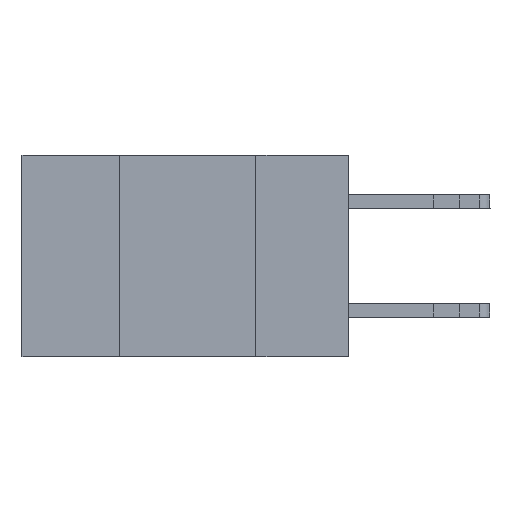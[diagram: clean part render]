
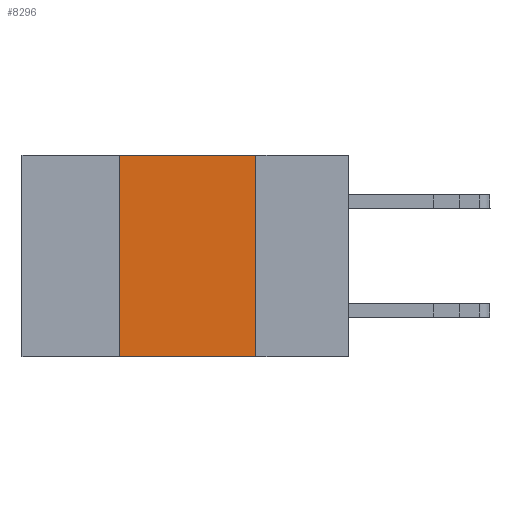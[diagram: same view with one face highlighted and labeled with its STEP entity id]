
A CAD part, left-side view. The second image highlights one B-rep face of the part: STEP entity #8296.
In plain terms, the highlighted planar face has unit normal (-1, 0, 0).
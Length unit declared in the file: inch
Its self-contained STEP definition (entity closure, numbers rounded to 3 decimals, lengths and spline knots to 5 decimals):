
#655 = CARTESIAN_POINT ( 'NONE',  ( 0., 0.6, 0. ) ) ;
#1183 = ORIENTED_EDGE ( 'NONE', *, *, #12697, .T. ) ;
#1598 = DIRECTION ( 'NONE',  ( 1., 0., 0. ) ) ;
#2758 = LINE ( 'NONE', #12832, #5205 ) ;
#3607 = LINE ( 'NONE', #655, #8730 ) ;
#3857 = ORIENTED_EDGE ( 'NONE', *, *, #12679, .F. ) ;
#4478 = CARTESIAN_POINT ( 'NONE',  ( 0., 0.42, -0.37 ) ) ;
#4522 = CARTESIAN_POINT ( 'NONE',  ( 0., 0.42, -0.37 ) ) ;
#4604 = CARTESIAN_POINT ( 'NONE',  ( 0., 0.6, 0. ) ) ;
#4645 = DIRECTION ( 'NONE',  ( 0., -1., 0. ) ) ;
#4811 = EDGE_CURVE ( 'NONE', #7847, #6638, #12779, .T. ) ;
#5205 = VECTOR ( 'NONE', #12702, 39.37008 ) ;
#5540 = ORIENTED_EDGE ( 'NONE', *, *, #8302, .F. ) ;
#5702 = DIRECTION ( 'NONE',  ( 0., 0., -1. ) ) ;
#6638 = VERTEX_POINT ( 'NONE', #11011 ) ;
#6675 = CARTESIAN_POINT ( 'NONE',  ( 0., 0.17, -0.37 ) ) ;
#7478 = FACE_OUTER_BOUND ( 'NONE', #10889, .T. ) ;
#7738 = AXIS2_PLACEMENT_3D ( 'NONE', #4604, #1598, #12474 ) ;
#7847 = VERTEX_POINT ( 'NONE', #11649 ) ;
#7904 = VECTOR ( 'NONE', #5702, 39.37008 ) ;
#8296 = ADVANCED_FACE ( 'NONE', ( #7478 ), #10726, .F. ) ;
#8302 = EDGE_CURVE ( 'NONE', #10183, #9347, #9549, .T. ) ;
#8730 = VECTOR ( 'NONE', #4645, 39.37008 ) ;
#9347 = VERTEX_POINT ( 'NONE', #10995 ) ;
#9549 = LINE ( 'NONE', #4478, #11277 ) ;
#10183 = VERTEX_POINT ( 'NONE', #4522 ) ;
#10726 = PLANE ( 'NONE',  #7738 ) ;
#10889 = EDGE_LOOP ( 'NONE', ( #12692, #3857, #5540, #1183 ) ) ;
#10995 = CARTESIAN_POINT ( 'NONE',  ( 0., 0.42, 0. ) ) ;
#11011 = CARTESIAN_POINT ( 'NONE',  ( 0., 0.17, -0.37 ) ) ;
#11277 = VECTOR ( 'NONE', #11702, 39.37008 ) ;
#11649 = CARTESIAN_POINT ( 'NONE',  ( 0., 0.17, 0. ) ) ;
#11702 = DIRECTION ( 'NONE',  ( 0., 0., 1. ) ) ;
#12474 = DIRECTION ( 'NONE',  ( 0., 0., -1. ) ) ;
#12679 = EDGE_CURVE ( 'NONE', #9347, #7847, #3607, .T. ) ;
#12692 = ORIENTED_EDGE ( 'NONE', *, *, #4811, .F. ) ;
#12697 = EDGE_CURVE ( 'NONE', #10183, #6638, #2758, .T. ) ;
#12702 = DIRECTION ( 'NONE',  ( 0., -1., 0. ) ) ;
#12779 = LINE ( 'NONE', #6675, #7904 ) ;
#12832 = CARTESIAN_POINT ( 'NONE',  ( 0., 0.6, -0.37 ) ) ;
